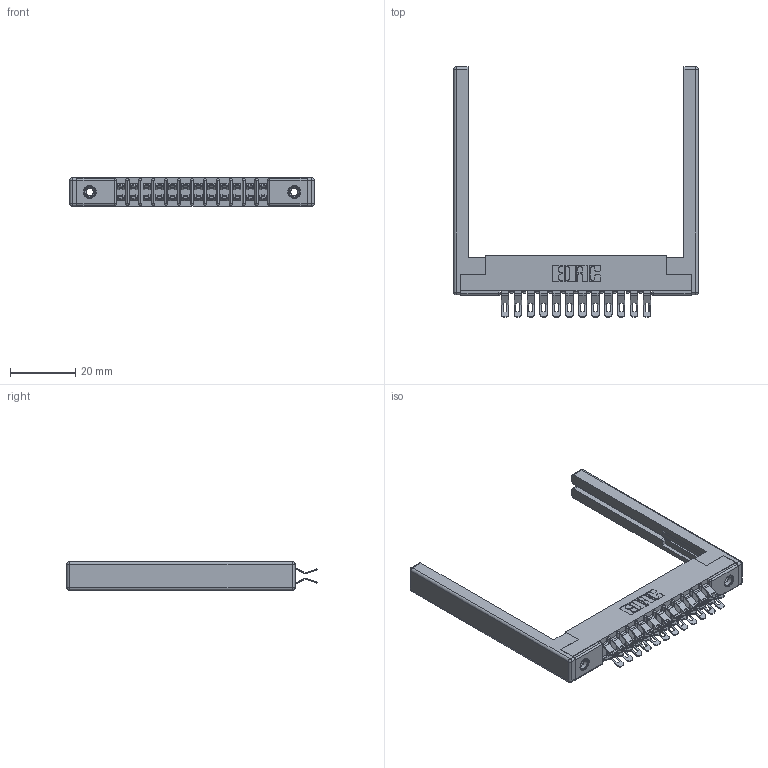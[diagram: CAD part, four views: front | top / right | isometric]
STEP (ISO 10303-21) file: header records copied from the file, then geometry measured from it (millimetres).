
FILE_DESCRIPTION (( 'STEP AP203' ), '1' );
FILE_NAME ('307-024-555-268.STEP', '2019-09-05T22:19:31', ( '' ), ( '' ), 'SwSTEP 2.0', 'SolidWorks 2016', '' );
FILE_SCHEMA (( 'CONFIG_CONTROL_DESIGN' ));
Length unit declared in the file: inch
Products named in the file (5): 307-220-068; 307 Part_.156 Dia Mounting Holes; 345-250-001_345-250-001-102; 307-024-555-268; 307-290-001_555
Assembly tree (29 placements, depth 2):
  307-024-555-268
    307 Part_.156 Dia Mounting Holes
    307-290-001_555  x24
    307-220-068  x2
    345-250-001_345-250-001-102  x2
Bounding box: 74.98 x 76.71 x 8.71 mm (x, y, z)
Volume: 9538.7 mm3; surface area: 12708.3 mm2
Topology: 29 solids, 29 shells, 1749 faces, 5057 edges, 3282 vertices
Faces by surface type: plane 974, cylinder 725, sphere 34, cone 12, torus 4
Entity records: 17666 total; most frequent: CARTESIAN_POINT 2881, DIRECTION 2857, ORIENTED_EDGE 2846, EDGE_CURVE 1423, LINE 1065, VECTOR 1065, VERTEX_POINT 920, AXIS2_PLACEMENT_3D 896
